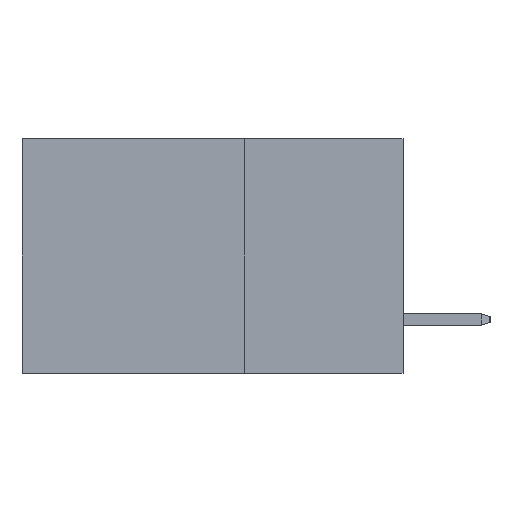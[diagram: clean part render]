
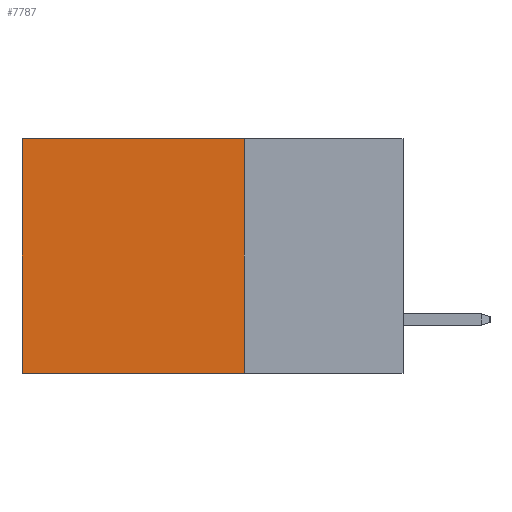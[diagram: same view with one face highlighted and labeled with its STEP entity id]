
A CAD part, left-side view. The second image highlights one B-rep face of the part: STEP entity #7787.
In plain terms, the highlighted planar face has unit normal (-1, 0, 0).
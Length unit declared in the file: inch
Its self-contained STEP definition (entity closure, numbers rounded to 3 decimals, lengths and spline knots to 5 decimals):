
#47 = CARTESIAN_POINT ( 'NONE',  ( 0.2875, 0.6, 0. ) ) ;
#477 = VECTOR ( 'NONE', #16366, 39.37008 ) ;
#1509 = DIRECTION ( 'NONE',  ( 0., 0., -1. ) ) ;
#1660 = LINE ( 'NONE', #16191, #17278 ) ;
#1969 = EDGE_CURVE ( 'NONE', #3371, #12458, #1660, .T. ) ;
#3371 = VERTEX_POINT ( 'NONE', #5701 ) ;
#3512 = DIRECTION ( 'NONE',  ( 0., 1., 0. ) ) ;
#3772 = VECTOR ( 'NONE', #1509, 39.37008 ) ;
#4473 = EDGE_CURVE ( 'NONE', #13165, #3371, #7913, .T. ) ;
#4854 = LINE ( 'NONE', #8170, #477 ) ;
#5390 = EDGE_CURVE ( 'NONE', #13165, #10747, #4854, .T. ) ;
#5701 = CARTESIAN_POINT ( 'NONE',  ( 0.2875, 0.25, -0.37 ) ) ;
#6193 = ORIENTED_EDGE ( 'NONE', *, *, #5390, .T. ) ;
#7327 = ORIENTED_EDGE ( 'NONE', *, *, #1969, .F. ) ;
#7787 = ADVANCED_FACE ( 'NONE', ( #17309 ), #16913, .F. ) ;
#7913 = LINE ( 'NONE', #12578, #10446 ) ;
#8170 = CARTESIAN_POINT ( 'NONE',  ( 0.2875, 0.25, 0. ) ) ;
#8584 = CARTESIAN_POINT ( 'NONE',  ( 0.2875, 0.6, -0.37 ) ) ;
#9112 = DIRECTION ( 'NONE',  ( 0., 0., -1. ) ) ;
#9915 = ORIENTED_EDGE ( 'NONE', *, *, #4473, .F. ) ;
#10175 = CARTESIAN_POINT ( 'NONE',  ( 0.2875, 0.25, 0. ) ) ;
#10446 = VECTOR ( 'NONE', #11018, 39.37008 ) ;
#10747 = VERTEX_POINT ( 'NONE', #18874 ) ;
#11018 = DIRECTION ( 'NONE',  ( 0., 0., -1. ) ) ;
#12458 = VERTEX_POINT ( 'NONE', #8584 ) ;
#12578 = CARTESIAN_POINT ( 'NONE',  ( 0.2875, 0.25, 0. ) ) ;
#13165 = VERTEX_POINT ( 'NONE', #10175 ) ;
#13581 = EDGE_LOOP ( 'NONE', ( #19232, #7327, #9915, #6193 ) ) ;
#13958 = AXIS2_PLACEMENT_3D ( 'NONE', #17009, #17120, #9112 ) ;
#16191 = CARTESIAN_POINT ( 'NONE',  ( 0.2875, 0.25, -0.37 ) ) ;
#16366 = DIRECTION ( 'NONE',  ( 0., 1., 0. ) ) ;
#16374 = EDGE_CURVE ( 'NONE', #10747, #12458, #19261, .T. ) ;
#16913 = PLANE ( 'NONE',  #13958 ) ;
#17009 = CARTESIAN_POINT ( 'NONE',  ( 0.2875, 0.25, 0. ) ) ;
#17120 = DIRECTION ( 'NONE',  ( 1., 0., 0. ) ) ;
#17278 = VECTOR ( 'NONE', #3512, 39.37008 ) ;
#17309 = FACE_OUTER_BOUND ( 'NONE', #13581, .T. ) ;
#18874 = CARTESIAN_POINT ( 'NONE',  ( 0.2875, 0.6, 0. ) ) ;
#19232 = ORIENTED_EDGE ( 'NONE', *, *, #16374, .T. ) ;
#19261 = LINE ( 'NONE', #47, #3772 ) ;
